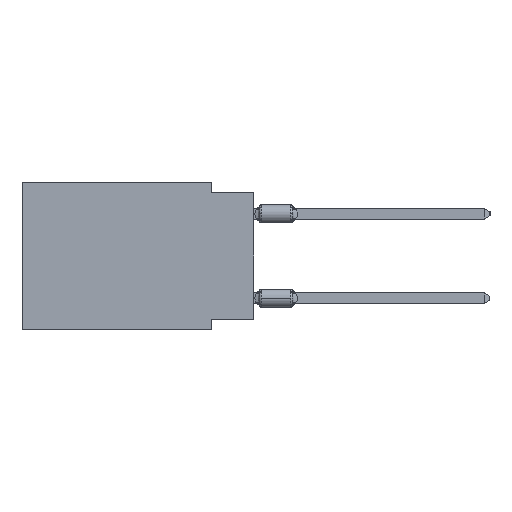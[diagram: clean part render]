
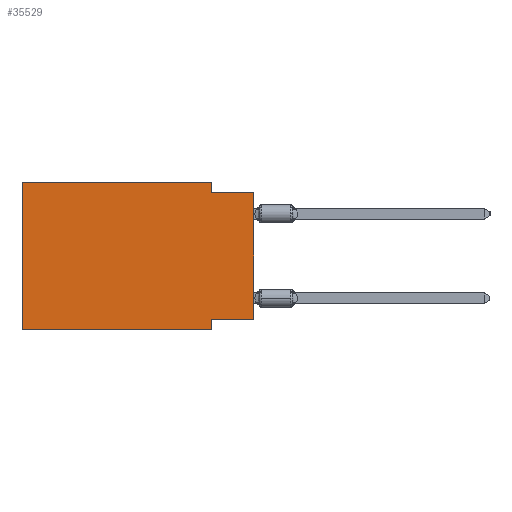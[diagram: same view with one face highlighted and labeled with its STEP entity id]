
A CAD part, left-side view. The second image highlights one B-rep face of the part: STEP entity #35529.
In plain terms, the highlighted planar face has unit normal (-1, 0, 0).
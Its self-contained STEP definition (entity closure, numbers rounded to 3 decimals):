
#1221 = VERTEX_POINT ( 'NONE', #38891 ) ;
#1391 = CARTESIAN_POINT ( 'NONE',  ( 0., 2.54, -8.89 ) ) ;
#1610 = DIRECTION ( 'NONE',  ( 0., 0., 1. ) ) ;
#2130 = CARTESIAN_POINT ( 'NONE',  ( 0., 2.54, 0. ) ) ;
#3254 = VERTEX_POINT ( 'NONE', #2130 ) ;
#4804 = LINE ( 'NONE', #30768, #24746 ) ;
#5265 = VERTEX_POINT ( 'NONE', #30379 ) ;
#5277 = LINE ( 'NONE', #30045, #9684 ) ;
#5781 = VERTEX_POINT ( 'NONE', #5811 ) ;
#5801 = EDGE_CURVE ( 'NONE', #5265, #3254, #15395, .T. ) ;
#5811 = CARTESIAN_POINT ( 'NONE',  ( 0., 13.97, -8.89 ) ) ;
#6181 = DIRECTION ( 'NONE',  ( 0., 0., -1. ) ) ;
#6231 = ORIENTED_EDGE ( 'NONE', *, *, #34855, .F. ) ;
#6520 = ORIENTED_EDGE ( 'NONE', *, *, #10449, .F. ) ;
#7569 = LINE ( 'NONE', #1391, #33237 ) ;
#8370 = VERTEX_POINT ( 'NONE', #30878 ) ;
#8569 = LINE ( 'NONE', #15160, #19782 ) ;
#8602 = DIRECTION ( 'NONE',  ( 0., -1., 0. ) ) ;
#9577 = CARTESIAN_POINT ( 'NONE',  ( 0., 13.97, 0. ) ) ;
#9684 = VECTOR ( 'NONE', #17055, 1000. ) ;
#10378 = VECTOR ( 'NONE', #26667, 1000. ) ;
#10449 = EDGE_CURVE ( 'NONE', #28633, #17369, #5277, .T. ) ;
#11375 = DIRECTION ( 'NONE',  ( 0., 0., -1. ) ) ;
#12521 = DIRECTION ( 'NONE',  ( 0., 0., -1. ) ) ;
#13668 = CARTESIAN_POINT ( 'NONE',  ( 0., 0., -0.635 ) ) ;
#15158 = ORIENTED_EDGE ( 'NONE', *, *, #31294, .T. ) ;
#15160 = CARTESIAN_POINT ( 'NONE',  ( 0., 0., 0. ) ) ;
#15395 = LINE ( 'NONE', #37727, #35320 ) ;
#16298 = CARTESIAN_POINT ( 'NONE',  ( 0., 2.54, -0.635 ) ) ;
#17055 = DIRECTION ( 'NONE',  ( 0., -1., 0. ) ) ;
#17369 = VERTEX_POINT ( 'NONE', #13668 ) ;
#17605 = ORIENTED_EDGE ( 'NONE', *, *, #21643, .F. ) ;
#18947 = FACE_OUTER_BOUND ( 'NONE', #38445, .T. ) ;
#19332 = CARTESIAN_POINT ( 'NONE',  ( 0., 2.54, 0. ) ) ;
#19575 = PLANE ( 'NONE',  #19837 ) ;
#19782 = VECTOR ( 'NONE', #28342, 1000. ) ;
#19837 = AXIS2_PLACEMENT_3D ( 'NONE', #9577, #32339, #6181 ) ;
#20058 = CARTESIAN_POINT ( 'NONE',  ( 0., 0., -8.255 ) ) ;
#21177 = EDGE_CURVE ( 'NONE', #5781, #33276, #24561, .T. ) ;
#21643 = EDGE_CURVE ( 'NONE', #5781, #5265, #4804, .T. ) ;
#21910 = CARTESIAN_POINT ( 'NONE',  ( 0., 2.54, -8.89 ) ) ;
#21994 = VECTOR ( 'NONE', #31558, 1000. ) ;
#24561 = LINE ( 'NONE', #31147, #21994 ) ;
#24746 = VECTOR ( 'NONE', #1610, 1000. ) ;
#26352 = LINE ( 'NONE', #19332, #31568 ) ;
#26667 = DIRECTION ( 'NONE',  ( 0., 1., 0. ) ) ;
#28134 = ORIENTED_EDGE ( 'NONE', *, *, #41398, .F. ) ;
#28342 = DIRECTION ( 'NONE',  ( 0., 0., 1. ) ) ;
#28633 = VERTEX_POINT ( 'NONE', #16298 ) ;
#30045 = CARTESIAN_POINT ( 'NONE',  ( 0., 0., -0.635 ) ) ;
#30379 = CARTESIAN_POINT ( 'NONE',  ( 0., 13.97, 0. ) ) ;
#30768 = CARTESIAN_POINT ( 'NONE',  ( 0., 13.97, 0. ) ) ;
#30876 = ORIENTED_EDGE ( 'NONE', *, *, #36448, .F. ) ;
#30878 = CARTESIAN_POINT ( 'NONE',  ( 0., 2.54, -8.255 ) ) ;
#31147 = CARTESIAN_POINT ( 'NONE',  ( 0., 13.97, -8.89 ) ) ;
#31294 = EDGE_CURVE ( 'NONE', #1221, #17369, #8569, .T. ) ;
#31558 = DIRECTION ( 'NONE',  ( 0., -1., 0. ) ) ;
#31568 = VECTOR ( 'NONE', #12521, 1000. ) ;
#32339 = DIRECTION ( 'NONE',  ( 1., 0., 0. ) ) ;
#32614 = ORIENTED_EDGE ( 'NONE', *, *, #5801, .F. ) ;
#32674 = ORIENTED_EDGE ( 'NONE', *, *, #21177, .T. ) ;
#33237 = VECTOR ( 'NONE', #11375, 1000. ) ;
#33276 = VERTEX_POINT ( 'NONE', #21910 ) ;
#34855 = EDGE_CURVE ( 'NONE', #8370, #33276, #7569, .T. ) ;
#35320 = VECTOR ( 'NONE', #8602, 1000. ) ;
#35529 = ADVANCED_FACE ( 'NONE', ( #18947 ), #19575, .F. ) ;
#36448 = EDGE_CURVE ( 'NONE', #1221, #8370, #37060, .T. ) ;
#37060 = LINE ( 'NONE', #20058, #10378 ) ;
#37727 = CARTESIAN_POINT ( 'NONE',  ( 0., 13.97, 0. ) ) ;
#38445 = EDGE_LOOP ( 'NONE', ( #15158, #6520, #28134, #32614, #17605, #32674, #6231, #30876 ) ) ;
#38891 = CARTESIAN_POINT ( 'NONE',  ( 0., 0., -8.255 ) ) ;
#41398 = EDGE_CURVE ( 'NONE', #3254, #28633, #26352, .T. ) ;
